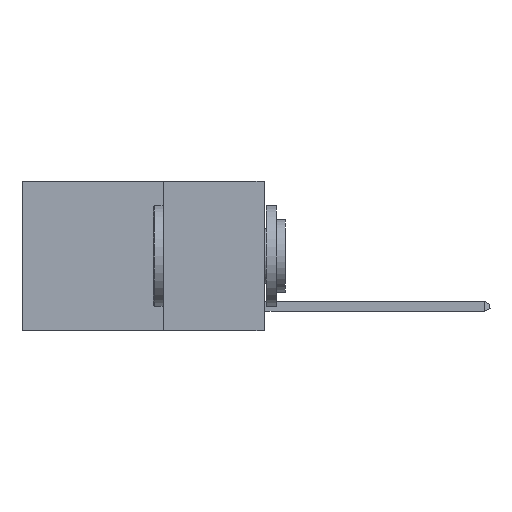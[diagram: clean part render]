
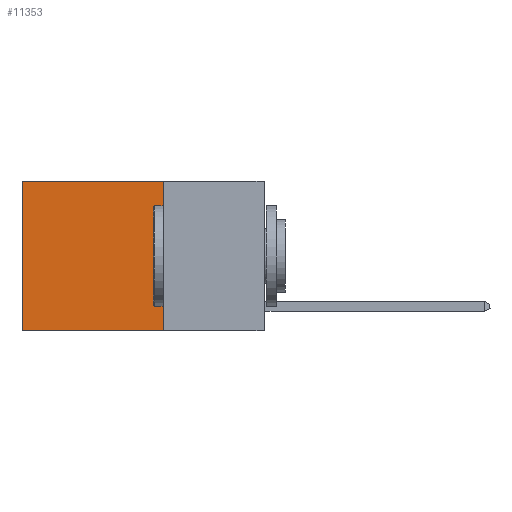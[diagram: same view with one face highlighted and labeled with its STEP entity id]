
A CAD part, left-side view. The second image highlights one B-rep face of the part: STEP entity #11353.
In plain terms, the highlighted planar face has unit normal (-1, 0, 0).
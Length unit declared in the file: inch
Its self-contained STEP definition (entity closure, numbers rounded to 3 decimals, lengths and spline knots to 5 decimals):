
#407 = VECTOR ( 'NONE', #3821, 39.37008 ) ;
#2007 = DIRECTION ( 'NONE',  ( 1., 0., 0. ) ) ;
#2747 = CARTESIAN_POINT ( 'NONE',  ( 0.2625, 0.25, -0.37 ) ) ;
#3546 = EDGE_CURVE ( 'NONE', #14938, #13351, #14489, .T. ) ;
#3819 = CARTESIAN_POINT ( 'NONE',  ( 0.2625, 0.25, -0.37 ) ) ;
#3821 = DIRECTION ( 'NONE',  ( 0., 1., 0. ) ) ;
#4372 = CARTESIAN_POINT ( 'NONE',  ( 0.2625, 0.25, 0. ) ) ;
#4751 = CARTESIAN_POINT ( 'NONE',  ( 0.2625, 0.25, 0. ) ) ;
#5342 = VECTOR ( 'NONE', #10772, 39.37008 ) ;
#5671 = DIRECTION ( 'NONE',  ( 0., 0., -1. ) ) ;
#6212 = CARTESIAN_POINT ( 'NONE',  ( 0.2625, 0.6, 0. ) ) ;
#6306 = EDGE_LOOP ( 'NONE', ( #9786, #6960, #13286, #6705 ) ) ;
#6705 = ORIENTED_EDGE ( 'NONE', *, *, #7250, .T. ) ;
#6755 = EDGE_CURVE ( 'NONE', #13351, #10608, #8969, .T. ) ;
#6960 = ORIENTED_EDGE ( 'NONE', *, *, #6755, .F. ) ;
#7250 = EDGE_CURVE ( 'NONE', #14938, #8774, #13478, .T. ) ;
#8411 = FACE_OUTER_BOUND ( 'NONE', #6306, .T. ) ;
#8774 = VERTEX_POINT ( 'NONE', #13320 ) ;
#8969 = LINE ( 'NONE', #2747, #407 ) ;
#9120 = AXIS2_PLACEMENT_3D ( 'NONE', #4372, #2007, #5671 ) ;
#9786 = ORIENTED_EDGE ( 'NONE', *, *, #10534, .T. ) ;
#9846 = CARTESIAN_POINT ( 'NONE',  ( 0.2625, 0.6, -0.37 ) ) ;
#10138 = VECTOR ( 'NONE', #12259, 39.37008 ) ;
#10534 = EDGE_CURVE ( 'NONE', #8774, #10608, #11126, .T. ) ;
#10608 = VERTEX_POINT ( 'NONE', #9846 ) ;
#10772 = DIRECTION ( 'NONE',  ( 0., 0., -1. ) ) ;
#11126 = LINE ( 'NONE', #6212, #11946 ) ;
#11353 = ADVANCED_FACE ( 'NONE', ( #8411 ), #13092, .F. ) ;
#11946 = VECTOR ( 'NONE', #13302, 39.37008 ) ;
#12259 = DIRECTION ( 'NONE',  ( 0., 1., 0. ) ) ;
#13092 = PLANE ( 'NONE',  #9120 ) ;
#13286 = ORIENTED_EDGE ( 'NONE', *, *, #3546, .F. ) ;
#13302 = DIRECTION ( 'NONE',  ( 0., 0., -1. ) ) ;
#13320 = CARTESIAN_POINT ( 'NONE',  ( 0.2625, 0.6, 0. ) ) ;
#13351 = VERTEX_POINT ( 'NONE', #3819 ) ;
#13478 = LINE ( 'NONE', #15021, #10138 ) ;
#14489 = LINE ( 'NONE', #15550, #5342 ) ;
#14938 = VERTEX_POINT ( 'NONE', #4751 ) ;
#15021 = CARTESIAN_POINT ( 'NONE',  ( 0.2625, 0.25, 0. ) ) ;
#15550 = CARTESIAN_POINT ( 'NONE',  ( 0.2625, 0.25, 0. ) ) ;
